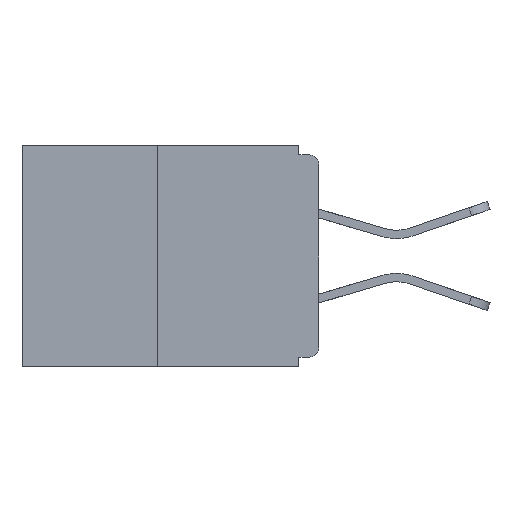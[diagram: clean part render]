
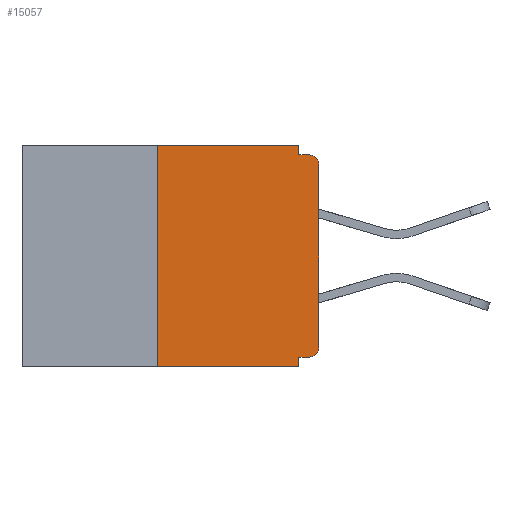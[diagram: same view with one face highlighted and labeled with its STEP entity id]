
A CAD part, left-side view. The second image highlights one B-rep face of the part: STEP entity #15057.
In plain terms, the highlighted planar face has unit normal (-1, 0, 0).
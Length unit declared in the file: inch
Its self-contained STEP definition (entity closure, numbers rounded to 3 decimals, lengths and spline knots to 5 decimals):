
#619 = CARTESIAN_POINT ( 'NONE',  ( 0., 0.015, -0.03 ) ) ;
#696 = VECTOR ( 'NONE', #3985, 39.37008 ) ;
#753 = ORIENTED_EDGE ( 'NONE', *, *, #11044, .T. ) ;
#839 = VERTEX_POINT ( 'NONE', #11449 ) ;
#856 = EDGE_CURVE ( 'NONE', #8677, #10585, #12946, .T. ) ;
#1054 = EDGE_CURVE ( 'NONE', #9454, #5364, #7737, .T. ) ;
#1182 = CARTESIAN_POINT ( 'NONE',  ( 0., 0.031, -0.328 ) ) ;
#1326 = ORIENTED_EDGE ( 'NONE', *, *, #6608, .F. ) ;
#1467 = VERTEX_POINT ( 'NONE', #11282 ) ;
#1529 = EDGE_CURVE ( 'NONE', #9454, #8579, #2127, .T. ) ;
#1614 = DIRECTION ( 'NONE',  ( 0., 0., -1. ) ) ;
#1674 = CARTESIAN_POINT ( 'NONE',  ( 0., 0., -0.03 ) ) ;
#2078 = DIRECTION ( 'NONE',  ( 0., -1., 0. ) ) ;
#2127 = LINE ( 'NONE', #8023, #6040 ) ;
#2934 = EDGE_LOOP ( 'NONE', ( #5786, #6626, #15047, #4434, #5462, #753, #4089, #10073, #3858, #1326 ) ) ;
#3033 = VECTOR ( 'NONE', #6084, 39.37008 ) ;
#3218 = CARTESIAN_POINT ( 'NONE',  ( 0., 0.46, 0. ) ) ;
#3858 = ORIENTED_EDGE ( 'NONE', *, *, #6298, .F. ) ;
#3985 = DIRECTION ( 'NONE',  ( 0., 0., 1. ) ) ;
#4089 = ORIENTED_EDGE ( 'NONE', *, *, #8295, .T. ) ;
#4434 = ORIENTED_EDGE ( 'NONE', *, *, #5783, .F. ) ;
#4591 = CARTESIAN_POINT ( 'NONE',  ( 0., 0., -0.015 ) ) ;
#4625 = VERTEX_POINT ( 'NONE', #9708 ) ;
#4680 = DIRECTION ( 'NONE',  ( -1., 0., 0. ) ) ;
#5302 = DIRECTION ( 'NONE',  ( 0., 1., 0. ) ) ;
#5364 = VERTEX_POINT ( 'NONE', #9592 ) ;
#5462 = ORIENTED_EDGE ( 'NONE', *, *, #6877, .F. ) ;
#5783 = EDGE_CURVE ( 'NONE', #10918, #8579, #11971, .T. ) ;
#5786 = ORIENTED_EDGE ( 'NONE', *, *, #14962, .F. ) ;
#5806 = CARTESIAN_POINT ( 'NONE',  ( 0., 0.015, -0.313 ) ) ;
#5995 = VECTOR ( 'NONE', #12940, 39.37008 ) ;
#6040 = VECTOR ( 'NONE', #2078, 39.37008 ) ;
#6084 = DIRECTION ( 'NONE',  ( 0., 0., -1. ) ) ;
#6298 = EDGE_CURVE ( 'NONE', #4625, #10585, #7110, .T. ) ;
#6558 = CARTESIAN_POINT ( 'NONE',  ( 0., 0.46, 0. ) ) ;
#6608 = EDGE_CURVE ( 'NONE', #9421, #4625, #8762, .T. ) ;
#6626 = ORIENTED_EDGE ( 'NONE', *, *, #1054, .F. ) ;
#6722 = LINE ( 'NONE', #12339, #9127 ) ;
#6756 = DIRECTION ( 'NONE',  ( 1., 0., 0. ) ) ;
#6800 = DIRECTION ( 'NONE',  ( 0., 0., -1. ) ) ;
#6877 = EDGE_CURVE ( 'NONE', #839, #10918, #6722, .T. ) ;
#7102 = AXIS2_PLACEMENT_3D ( 'NONE', #5806, #4680, #12816 ) ;
#7110 = LINE ( 'NONE', #4591, #5995 ) ;
#7198 = CARTESIAN_POINT ( 'NONE',  ( 0., 0.25, -0.343 ) ) ;
#7656 = VECTOR ( 'NONE', #10268, 39.37008 ) ;
#7737 = LINE ( 'NONE', #8628, #696 ) ;
#8023 = CARTESIAN_POINT ( 'NONE',  ( 0., 0.46, -0.343 ) ) ;
#8295 = EDGE_CURVE ( 'NONE', #1467, #8677, #8546, .T. ) ;
#8507 = CARTESIAN_POINT ( 'NONE',  ( 0., 0.031, 0. ) ) ;
#8546 = LINE ( 'NONE', #14143, #13350 ) ;
#8579 = VERTEX_POINT ( 'NONE', #10044 ) ;
#8628 = CARTESIAN_POINT ( 'NONE',  ( 0., 0.25, 0. ) ) ;
#8677 = VERTEX_POINT ( 'NONE', #1674 ) ;
#8742 = DIRECTION ( 'NONE',  ( -1., 0., 0. ) ) ;
#8762 = LINE ( 'NONE', #14845, #7656 ) ;
#9127 = VECTOR ( 'NONE', #5302, 39.37008 ) ;
#9421 = VERTEX_POINT ( 'NONE', #8507 ) ;
#9454 = VERTEX_POINT ( 'NONE', #7198 ) ;
#9592 = CARTESIAN_POINT ( 'NONE',  ( 0., 0.25, 0. ) ) ;
#9708 = CARTESIAN_POINT ( 'NONE',  ( 0., 0.031, -0.015 ) ) ;
#9812 = CARTESIAN_POINT ( 'NONE',  ( 0., 0.031, -0.343 ) ) ;
#10044 = CARTESIAN_POINT ( 'NONE',  ( 0., 0.031, -0.343 ) ) ;
#10073 = ORIENTED_EDGE ( 'NONE', *, *, #856, .T. ) ;
#10268 = DIRECTION ( 'NONE',  ( 0., 0., -1. ) ) ;
#10585 = VERTEX_POINT ( 'NONE', #10636 ) ;
#10636 = CARTESIAN_POINT ( 'NONE',  ( 0., 0.015, -0.015 ) ) ;
#10918 = VERTEX_POINT ( 'NONE', #1182 ) ;
#11044 = EDGE_CURVE ( 'NONE', #839, #1467, #14645, .T. ) ;
#11282 = CARTESIAN_POINT ( 'NONE',  ( 0., 0., -0.313 ) ) ;
#11449 = CARTESIAN_POINT ( 'NONE',  ( 0., 0.015, -0.328 ) ) ;
#11464 = AXIS2_PLACEMENT_3D ( 'NONE', #619, #8742, #1614 ) ;
#11971 = LINE ( 'NONE', #9812, #3033 ) ;
#12339 = CARTESIAN_POINT ( 'NONE',  ( 0., 0., -0.328 ) ) ;
#12674 = DIRECTION ( 'NONE',  ( 0., -1., 0. ) ) ;
#12816 = DIRECTION ( 'NONE',  ( 0., 0., -1. ) ) ;
#12859 = VECTOR ( 'NONE', #12674, 39.37008 ) ;
#12940 = DIRECTION ( 'NONE',  ( 0., -1., 0. ) ) ;
#12946 = CIRCLE ( 'NONE', #11464, 0.015 ) ;
#13324 = AXIS2_PLACEMENT_3D ( 'NONE', #3218, #6756, #6800 ) ;
#13350 = VECTOR ( 'NONE', #15331, 39.37008 ) ;
#13591 = FACE_OUTER_BOUND ( 'NONE', #2934, .T. ) ;
#13852 = PLANE ( 'NONE',  #13324 ) ;
#14143 = CARTESIAN_POINT ( 'NONE',  ( 0., 0., 0. ) ) ;
#14645 = CIRCLE ( 'NONE', #7102, 0.015 ) ;
#14845 = CARTESIAN_POINT ( 'NONE',  ( 0., 0.031, 0. ) ) ;
#14962 = EDGE_CURVE ( 'NONE', #5364, #9421, #15100, .T. ) ;
#15047 = ORIENTED_EDGE ( 'NONE', *, *, #1529, .T. ) ;
#15057 = ADVANCED_FACE ( 'NONE', ( #13591 ), #13852, .F. ) ;
#15100 = LINE ( 'NONE', #6558, #12859 ) ;
#15331 = DIRECTION ( 'NONE',  ( 0., 0., 1. ) ) ;
